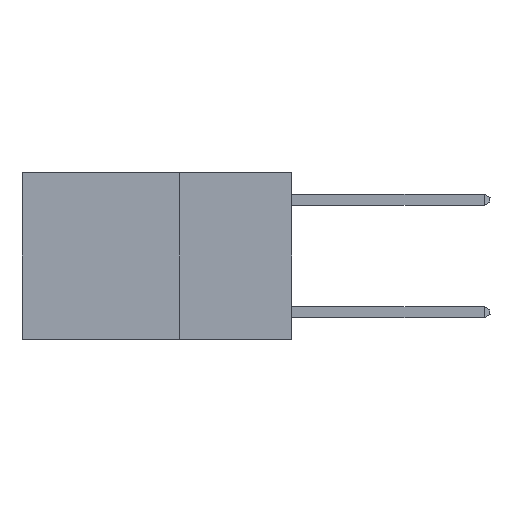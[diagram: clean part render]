
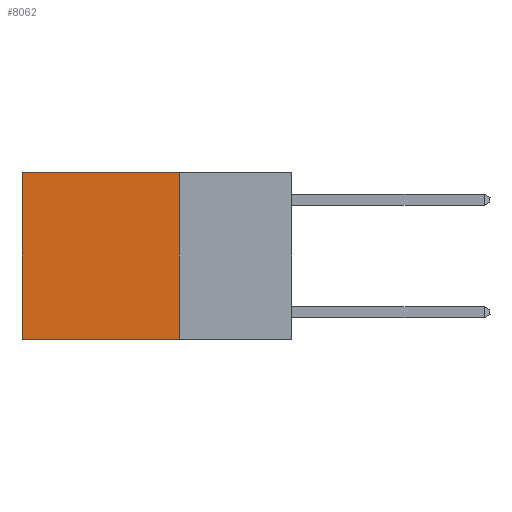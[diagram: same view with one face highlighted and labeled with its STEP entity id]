
A CAD part, left-side view. The second image highlights one B-rep face of the part: STEP entity #8062.
In plain terms, the highlighted planar face has unit normal (-1, 0, 0).
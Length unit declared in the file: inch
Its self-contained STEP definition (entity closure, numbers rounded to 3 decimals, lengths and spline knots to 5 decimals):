
#1415 = DIRECTION ( 'NONE',  ( 1., 0., 0. ) ) ;
#1595 = VERTEX_POINT ( 'NONE', #6696 ) ;
#2615 = CARTESIAN_POINT ( 'NONE',  ( 0.2625, 0.6, 0. ) ) ;
#3634 = EDGE_CURVE ( 'NONE', #6740, #11733, #5839, .T. ) ;
#3992 = CARTESIAN_POINT ( 'NONE',  ( 0.2625, 0.25, -0.37 ) ) ;
#5134 = EDGE_CURVE ( 'NONE', #1595, #6740, #10435, .T. ) ;
#5193 = ORIENTED_EDGE ( 'NONE', *, *, #12075, .F. ) ;
#5691 = EDGE_LOOP ( 'NONE', ( #12024, #10372, #5193, #6410 ) ) ;
#5839 = LINE ( 'NONE', #10365, #7202 ) ;
#5921 = DIRECTION ( 'NONE',  ( 0., 0., -1. ) ) ;
#6410 = ORIENTED_EDGE ( 'NONE', *, *, #5134, .T. ) ;
#6696 = CARTESIAN_POINT ( 'NONE',  ( 0.2625, 0.25, 0. ) ) ;
#6740 = VERTEX_POINT ( 'NONE', #2615 ) ;
#7202 = VECTOR ( 'NONE', #15083, 39.37008 ) ;
#7239 = PLANE ( 'NONE',  #9492 ) ;
#7463 = VECTOR ( 'NONE', #12291, 39.37008 ) ;
#7529 = CARTESIAN_POINT ( 'NONE',  ( 0.2625, 0.6, -0.37 ) ) ;
#8062 = ADVANCED_FACE ( 'NONE', ( #11617 ), #7239, .F. ) ;
#8907 = CARTESIAN_POINT ( 'NONE',  ( 0.2625, 0.25, 0. ) ) ;
#9492 = AXIS2_PLACEMENT_3D ( 'NONE', #11765, #1415, #5921 ) ;
#10365 = CARTESIAN_POINT ( 'NONE',  ( 0.2625, 0.6, 0. ) ) ;
#10372 = ORIENTED_EDGE ( 'NONE', *, *, #10872, .F. ) ;
#10435 = LINE ( 'NONE', #8907, #7463 ) ;
#10511 = VECTOR ( 'NONE', #12185, 39.37008 ) ;
#10872 = EDGE_CURVE ( 'NONE', #14531, #11733, #13747, .T. ) ;
#11019 = VECTOR ( 'NONE', #14389, 39.37008 ) ;
#11617 = FACE_OUTER_BOUND ( 'NONE', #5691, .T. ) ;
#11733 = VERTEX_POINT ( 'NONE', #7529 ) ;
#11765 = CARTESIAN_POINT ( 'NONE',  ( 0.2625, 0.25, 0. ) ) ;
#12024 = ORIENTED_EDGE ( 'NONE', *, *, #3634, .T. ) ;
#12075 = EDGE_CURVE ( 'NONE', #1595, #14531, #12114, .T. ) ;
#12114 = LINE ( 'NONE', #13120, #11019 ) ;
#12185 = DIRECTION ( 'NONE',  ( 0., 1., 0. ) ) ;
#12291 = DIRECTION ( 'NONE',  ( 0., 1., 0. ) ) ;
#13120 = CARTESIAN_POINT ( 'NONE',  ( 0.2625, 0.25, 0. ) ) ;
#13432 = CARTESIAN_POINT ( 'NONE',  ( 0.2625, 0.25, -0.37 ) ) ;
#13747 = LINE ( 'NONE', #13432, #10511 ) ;
#14389 = DIRECTION ( 'NONE',  ( 0., 0., -1. ) ) ;
#14531 = VERTEX_POINT ( 'NONE', #3992 ) ;
#15083 = DIRECTION ( 'NONE',  ( 0., 0., -1. ) ) ;
